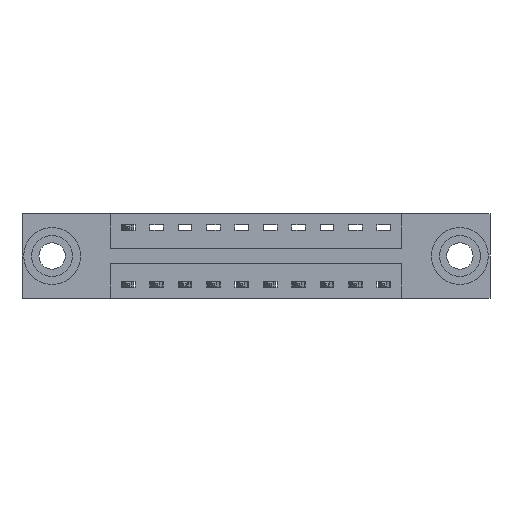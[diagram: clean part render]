
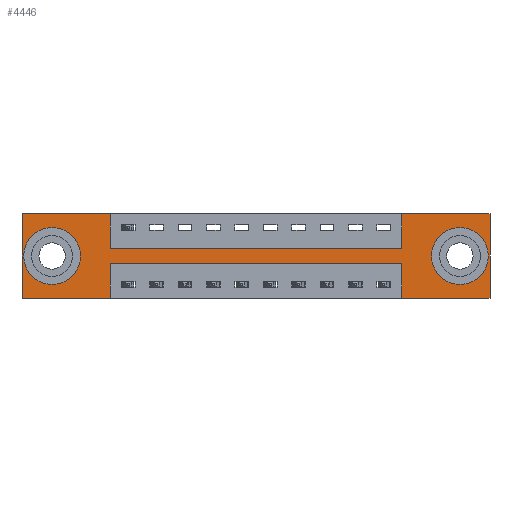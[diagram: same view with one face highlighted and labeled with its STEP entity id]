
A CAD part, front view. The second image highlights one B-rep face of the part: STEP entity #4446.
In plain terms, the highlighted planar face has unit normal (0, -1, 0).
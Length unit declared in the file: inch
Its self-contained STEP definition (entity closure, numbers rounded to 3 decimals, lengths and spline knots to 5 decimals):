
#37 = LINE ( 'NONE', #3687, #4768 ) ;
#526 = EDGE_CURVE ( 'NONE', #9319, #3657, #1531, .T. ) ;
#546 = CARTESIAN_POINT ( 'NONE',  ( 1.6725, 0., -0.37 ) ) ;
#667 = VECTOR ( 'NONE', #9513, 39.37008 ) ;
#686 = EDGE_CURVE ( 'NONE', #8400, #8053, #1926, .T. ) ;
#742 = DIRECTION ( 'NONE',  ( 0., 0., -1. ) ) ;
#768 = CARTESIAN_POINT ( 'NONE',  ( 1.6725, 0., 0. ) ) ;
#898 = CARTESIAN_POINT ( 'NONE',  ( 1.9275, 0., -0.185 ) ) ;
#1007 = ORIENTED_EDGE ( 'NONE', *, *, #7781, .F. ) ;
#1098 = CIRCLE ( 'NONE', #5388, 0.078 ) ;
#1147 = CARTESIAN_POINT ( 'NONE',  ( 0., 0., 0. ) ) ;
#1268 = ORIENTED_EDGE ( 'NONE', *, *, #3673, .F. ) ;
#1479 = VERTEX_POINT ( 'NONE', #1874 ) ;
#1508 = CARTESIAN_POINT ( 'NONE',  ( 0.1325, 0., -0.185 ) ) ;
#1531 = LINE ( 'NONE', #8769, #8385 ) ;
#1565 = CARTESIAN_POINT ( 'NONE',  ( 1.6725, 0., -0.37 ) ) ;
#1656 = VECTOR ( 'NONE', #4248, 39.37008 ) ;
#1657 = VECTOR ( 'NONE', #10104, 39.37008 ) ;
#1710 = LINE ( 'NONE', #2132, #10122 ) ;
#1755 = DIRECTION ( 'NONE',  ( 0., 0., -1. ) ) ;
#1765 = CARTESIAN_POINT ( 'NONE',  ( 0., 0., 0. ) ) ;
#1810 = ORIENTED_EDGE ( 'NONE', *, *, #9858, .F. ) ;
#1823 = CARTESIAN_POINT ( 'NONE',  ( 0.3875, 0., -0.15 ) ) ;
#1874 = CARTESIAN_POINT ( 'NONE',  ( 0.3875, 0., -0.37 ) ) ;
#1926 = LINE ( 'NONE', #546, #1656 ) ;
#1945 = VECTOR ( 'NONE', #9754, 39.37008 ) ;
#1997 = CARTESIAN_POINT ( 'NONE',  ( 2.06, 0., 0. ) ) ;
#2075 = ORIENTED_EDGE ( 'NONE', *, *, #2761, .F. ) ;
#2132 = CARTESIAN_POINT ( 'NONE',  ( 1.6725, 0., 0. ) ) ;
#2400 = DIRECTION ( 'NONE',  ( 0., 0., 1. ) ) ;
#2402 = EDGE_LOOP ( 'NONE', ( #3089, #5482 ) ) ;
#2761 = EDGE_CURVE ( 'NONE', #1479, #7886, #3029, .T. ) ;
#2856 = CARTESIAN_POINT ( 'NONE',  ( 0., 0., -0.37 ) ) ;
#2986 = DIRECTION ( 'NONE',  ( -1., 0., 0. ) ) ;
#3029 = LINE ( 'NONE', #3878, #5143 ) ;
#3032 = FACE_OUTER_BOUND ( 'NONE', #4127, .T. ) ;
#3089 = ORIENTED_EDGE ( 'NONE', *, *, #11057, .T. ) ;
#3263 = EDGE_CURVE ( 'NONE', #7886, #9319, #8463, .T. ) ;
#3264 = CIRCLE ( 'NONE', #10884, 0.078 ) ;
#3270 = VERTEX_POINT ( 'NONE', #1997 ) ;
#3641 = ORIENTED_EDGE ( 'NONE', *, *, #3932, .F. ) ;
#3657 = VERTEX_POINT ( 'NONE', #10646 ) ;
#3673 = EDGE_CURVE ( 'NONE', #6519, #8400, #8716, .T. ) ;
#3687 = CARTESIAN_POINT ( 'NONE',  ( 0.3875, 0., -0.37 ) ) ;
#3694 = VECTOR ( 'NONE', #9072, 39.37008 ) ;
#3878 = CARTESIAN_POINT ( 'NONE',  ( 0., 0., -0.37 ) ) ;
#3932 = EDGE_CURVE ( 'NONE', #3270, #6519, #7787, .T. ) ;
#3946 = CARTESIAN_POINT ( 'NONE',  ( 2.06, 0., -0.37 ) ) ;
#4127 = EDGE_LOOP ( 'NONE', ( #10045, #1007, #8129, #1268, #3641, #10540, #6353, #10798, #1810, #4208, #6647, #2075 ) ) ;
#4183 = CIRCLE ( 'NONE', #10399, 0.078 ) ;
#4208 = ORIENTED_EDGE ( 'NONE', *, *, #526, .F. ) ;
#4230 = EDGE_CURVE ( 'NONE', #8277, #6742, #1710, .T. ) ;
#4248 = DIRECTION ( 'NONE',  ( 0., 0., 1. ) ) ;
#4346 = CARTESIAN_POINT ( 'NONE',  ( 1.9275, 0., -0.107 ) ) ;
#4446 = ADVANCED_FACE ( 'NONE', ( #7818, #8078, #3032 ), #7841, .T. ) ;
#4632 = LINE ( 'NONE', #8955, #1945 ) ;
#4730 = VERTEX_POINT ( 'NONE', #4813 ) ;
#4745 = CARTESIAN_POINT ( 'NONE',  ( 0.3875, 0., -0.22 ) ) ;
#4768 = VECTOR ( 'NONE', #5513, 39.37008 ) ;
#4813 = CARTESIAN_POINT ( 'NONE',  ( 1.9275, 0., -0.263 ) ) ;
#5049 = VERTEX_POINT ( 'NONE', #4346 ) ;
#5143 = VECTOR ( 'NONE', #2986, 39.37008 ) ;
#5188 = DIRECTION ( 'NONE',  ( 0., 1., 0. ) ) ;
#5193 = CARTESIAN_POINT ( 'NONE',  ( 2.06, 0., 0. ) ) ;
#5296 = CARTESIAN_POINT ( 'NONE',  ( 1.9275, 0., -0.185 ) ) ;
#5388 = AXIS2_PLACEMENT_3D ( 'NONE', #10323, #5188, #11129 ) ;
#5398 = CARTESIAN_POINT ( 'NONE',  ( 0.1325, 0., -0.107 ) ) ;
#5482 = ORIENTED_EDGE ( 'NONE', *, *, #6604, .T. ) ;
#5513 = DIRECTION ( 'NONE',  ( 0., 0., -1. ) ) ;
#5597 = VERTEX_POINT ( 'NONE', #6224 ) ;
#5720 = EDGE_CURVE ( 'NONE', #7835, #8277, #9964, .T. ) ;
#5780 = VECTOR ( 'NONE', #10382, 39.37008 ) ;
#6070 = LINE ( 'NONE', #9581, #5780 ) ;
#6101 = DIRECTION ( 'NONE',  ( 0., -1., 0. ) ) ;
#6189 = LINE ( 'NONE', #8566, #1657 ) ;
#6224 = CARTESIAN_POINT ( 'NONE',  ( 0.1325, 0., -0.263 ) ) ;
#6229 = DIRECTION ( 'NONE',  ( 0., 0., -1. ) ) ;
#6301 = VERTEX_POINT ( 'NONE', #5398 ) ;
#6353 = ORIENTED_EDGE ( 'NONE', *, *, #4230, .F. ) ;
#6519 = VERTEX_POINT ( 'NONE', #3946 ) ;
#6537 = DIRECTION ( 'NONE',  ( 0., 0., 1. ) ) ;
#6604 = EDGE_CURVE ( 'NONE', #5597, #6301, #3264, .T. ) ;
#6647 = ORIENTED_EDGE ( 'NONE', *, *, #3263, .F. ) ;
#6742 = VERTEX_POINT ( 'NONE', #768 ) ;
#6846 = CARTESIAN_POINT ( 'NONE',  ( 1.6725, 0., -0.15 ) ) ;
#7192 = DIRECTION ( 'NONE',  ( 0., 1., 0. ) ) ;
#7228 = CIRCLE ( 'NONE', #7247, 0.078 ) ;
#7231 = AXIS2_PLACEMENT_3D ( 'NONE', #10305, #6101, #742 ) ;
#7247 = AXIS2_PLACEMENT_3D ( 'NONE', #898, #7192, #1755 ) ;
#7615 = ORIENTED_EDGE ( 'NONE', *, *, #11202, .T. ) ;
#7649 = EDGE_CURVE ( 'NONE', #6742, #3270, #6070, .T. ) ;
#7781 = EDGE_CURVE ( 'NONE', #8053, #10513, #4632, .T. ) ;
#7787 = LINE ( 'NONE', #5193, #667 ) ;
#7793 = VECTOR ( 'NONE', #8951, 39.37008 ) ;
#7800 = DIRECTION ( 'NONE',  ( 0., 1., 0. ) ) ;
#7818 = FACE_BOUND ( 'NONE', #8601, .T. ) ;
#7835 = VERTEX_POINT ( 'NONE', #8983 ) ;
#7841 = PLANE ( 'NONE',  #7231 ) ;
#7886 = VERTEX_POINT ( 'NONE', #2856 ) ;
#8053 = VERTEX_POINT ( 'NONE', #9997 ) ;
#8078 = FACE_BOUND ( 'NONE', #2402, .T. ) ;
#8129 = ORIENTED_EDGE ( 'NONE', *, *, #686, .F. ) ;
#8277 = VERTEX_POINT ( 'NONE', #6846 ) ;
#8284 = CARTESIAN_POINT ( 'NONE',  ( 0., 0., -0.37 ) ) ;
#8385 = VECTOR ( 'NONE', #9157, 39.37008 ) ;
#8400 = VERTEX_POINT ( 'NONE', #1565 ) ;
#8417 = DIRECTION ( 'NONE',  ( 0., 0., 1. ) ) ;
#8463 = LINE ( 'NONE', #1147, #10605 ) ;
#8566 = CARTESIAN_POINT ( 'NONE',  ( 0.3875, 0., 0. ) ) ;
#8601 = EDGE_LOOP ( 'NONE', ( #7615, #9795 ) ) ;
#8716 = LINE ( 'NONE', #8284, #3694 ) ;
#8769 = CARTESIAN_POINT ( 'NONE',  ( 0., 0., 0. ) ) ;
#8951 = DIRECTION ( 'NONE',  ( 1., 0., 0. ) ) ;
#8955 = CARTESIAN_POINT ( 'NONE',  ( 0.3875, 0., -0.22 ) ) ;
#8983 = CARTESIAN_POINT ( 'NONE',  ( 0.3875, 0., -0.15 ) ) ;
#9072 = DIRECTION ( 'NONE',  ( -1., 0., 0. ) ) ;
#9157 = DIRECTION ( 'NONE',  ( 1., 0., 0. ) ) ;
#9319 = VERTEX_POINT ( 'NONE', #1765 ) ;
#9435 = EDGE_CURVE ( 'NONE', #10513, #1479, #37, .T. ) ;
#9513 = DIRECTION ( 'NONE',  ( 0., 0., -1. ) ) ;
#9581 = CARTESIAN_POINT ( 'NONE',  ( 0., 0., 0. ) ) ;
#9754 = DIRECTION ( 'NONE',  ( -1., 0., 0. ) ) ;
#9795 = ORIENTED_EDGE ( 'NONE', *, *, #10153, .T. ) ;
#9858 = EDGE_CURVE ( 'NONE', #3657, #7835, #6189, .T. ) ;
#9964 = LINE ( 'NONE', #1823, #7793 ) ;
#9997 = CARTESIAN_POINT ( 'NONE',  ( 1.6725, 0., -0.22 ) ) ;
#10045 = ORIENTED_EDGE ( 'NONE', *, *, #9435, .F. ) ;
#10104 = DIRECTION ( 'NONE',  ( 0., 0., -1. ) ) ;
#10122 = VECTOR ( 'NONE', #8417, 39.37008 ) ;
#10153 = EDGE_CURVE ( 'NONE', #4730, #5049, #4183, .T. ) ;
#10305 = CARTESIAN_POINT ( 'NONE',  ( 0., 0., -0.37 ) ) ;
#10323 = CARTESIAN_POINT ( 'NONE',  ( 0.1325, 0., -0.185 ) ) ;
#10382 = DIRECTION ( 'NONE',  ( 1., 0., 0. ) ) ;
#10399 = AXIS2_PLACEMENT_3D ( 'NONE', #5296, #11224, #6229 ) ;
#10513 = VERTEX_POINT ( 'NONE', #4745 ) ;
#10540 = ORIENTED_EDGE ( 'NONE', *, *, #7649, .F. ) ;
#10605 = VECTOR ( 'NONE', #6537, 39.37008 ) ;
#10646 = CARTESIAN_POINT ( 'NONE',  ( 0.3875, 0., 0. ) ) ;
#10798 = ORIENTED_EDGE ( 'NONE', *, *, #5720, .F. ) ;
#10884 = AXIS2_PLACEMENT_3D ( 'NONE', #1508, #7800, #2400 ) ;
#11057 = EDGE_CURVE ( 'NONE', #6301, #5597, #1098, .T. ) ;
#11129 = DIRECTION ( 'NONE',  ( 0., 0., 1. ) ) ;
#11202 = EDGE_CURVE ( 'NONE', #5049, #4730, #7228, .T. ) ;
#11224 = DIRECTION ( 'NONE',  ( 0., 1., 0. ) ) ;
